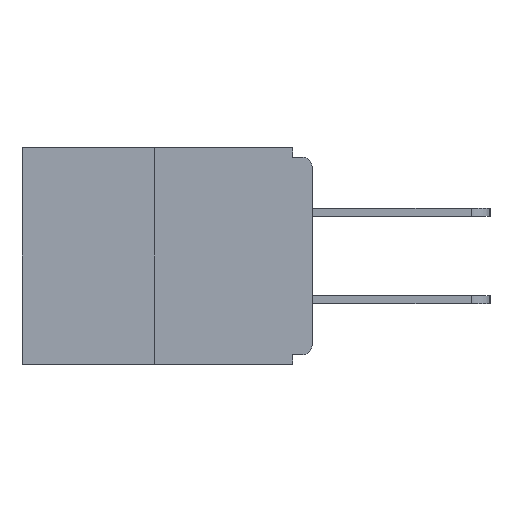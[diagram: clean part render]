
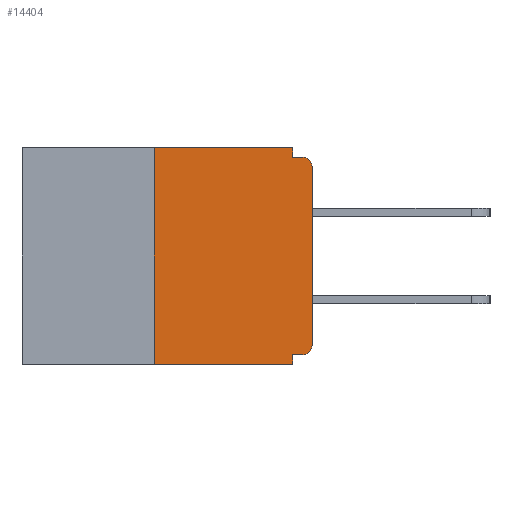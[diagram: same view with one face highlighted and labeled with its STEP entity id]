
A CAD part, left-side view. The second image highlights one B-rep face of the part: STEP entity #14404.
In plain terms, the highlighted planar face has unit normal (-1, 0, 0).
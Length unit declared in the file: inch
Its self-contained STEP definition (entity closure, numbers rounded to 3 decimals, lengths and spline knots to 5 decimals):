
#41 = LINE ( 'NONE', #24204, #22183 ) ;
#332 = DIRECTION ( 'NONE',  ( -1., 0., 0. ) ) ;
#713 = CARTESIAN_POINT ( 'NONE',  ( 0., 0.015, -0.03 ) ) ;
#792 = AXIS2_PLACEMENT_3D ( 'NONE', #713, #11689, #17690 ) ;
#1681 = VECTOR ( 'NONE', #19501, 39.37008 ) ;
#2002 = VERTEX_POINT ( 'NONE', #16268 ) ;
#2508 = PLANE ( 'NONE',  #15653 ) ;
#2662 = EDGE_CURVE ( 'NONE', #5712, #25853, #25253, .T. ) ;
#3229 = VECTOR ( 'NONE', #23539, 39.37008 ) ;
#3249 = CARTESIAN_POINT ( 'NONE',  ( 0., 0., -0.328 ) ) ;
#3826 = VECTOR ( 'NONE', #20638, 39.37008 ) ;
#4607 = LINE ( 'NONE', #23255, #6688 ) ;
#4760 = ORIENTED_EDGE ( 'NONE', *, *, #18055, .F. ) ;
#4921 = ORIENTED_EDGE ( 'NONE', *, *, #12934, .F. ) ;
#5234 = CARTESIAN_POINT ( 'NONE',  ( 0., 0.031, -0.015 ) ) ;
#5511 = FACE_OUTER_BOUND ( 'NONE', #9729, .T. ) ;
#5707 = CARTESIAN_POINT ( 'NONE',  ( 0., 0., -0.313 ) ) ;
#5712 = VERTEX_POINT ( 'NONE', #20174 ) ;
#5860 = VECTOR ( 'NONE', #27657, 39.37008 ) ;
#6462 = VERTEX_POINT ( 'NONE', #5234 ) ;
#6685 = EDGE_CURVE ( 'NONE', #16069, #20754, #12546, .T. ) ;
#6688 = VECTOR ( 'NONE', #21271, 39.37008 ) ;
#6735 = DIRECTION ( 'NONE',  ( 0., 0., -1. ) ) ;
#6820 = CARTESIAN_POINT ( 'NONE',  ( 0., 0.46, 0. ) ) ;
#6916 = DIRECTION ( 'NONE',  ( 1., 0., 0. ) ) ;
#7404 = CARTESIAN_POINT ( 'NONE',  ( 0., 0.25, 0. ) ) ;
#8445 = DIRECTION ( 'NONE',  ( 0., 0., 1. ) ) ;
#8929 = LINE ( 'NONE', #10278, #5860 ) ;
#9729 = EDGE_LOOP ( 'NONE', ( #18498, #25322, #17624, #4760, #11119, #21736, #12060, #12692, #4921, #25541 ) ) ;
#10278 = CARTESIAN_POINT ( 'NONE',  ( 0., 0.46, 0. ) ) ;
#10978 = EDGE_CURVE ( 'NONE', #5712, #16069, #27955, .T. ) ;
#11017 = VERTEX_POINT ( 'NONE', #11849 ) ;
#11119 = ORIENTED_EDGE ( 'NONE', *, *, #2662, .F. ) ;
#11344 = EDGE_CURVE ( 'NONE', #12639, #11017, #8929, .T. ) ;
#11689 = DIRECTION ( 'NONE',  ( -1., 0., 0. ) ) ;
#11849 = CARTESIAN_POINT ( 'NONE',  ( 0., 0.031, 0. ) ) ;
#11918 = EDGE_CURVE ( 'NONE', #12886, #14304, #26399, .T. ) ;
#12060 = ORIENTED_EDGE ( 'NONE', *, *, #6685, .T. ) ;
#12546 = LINE ( 'NONE', #21475, #22094 ) ;
#12639 = VERTEX_POINT ( 'NONE', #7404 ) ;
#12692 = ORIENTED_EDGE ( 'NONE', *, *, #19406, .T. ) ;
#12886 = VERTEX_POINT ( 'NONE', #19180 ) ;
#12934 = EDGE_CURVE ( 'NONE', #6462, #2002, #22286, .T. ) ;
#13142 = VECTOR ( 'NONE', #17829, 39.37008 ) ;
#13381 = CARTESIAN_POINT ( 'NONE',  ( 0., 0.015, -0.313 ) ) ;
#14304 = VERTEX_POINT ( 'NONE', #16043 ) ;
#14404 = ADVANCED_FACE ( 'NONE', ( #5511 ), #2508, .F. ) ;
#14409 = EDGE_CURVE ( 'NONE', #11017, #6462, #41, .T. ) ;
#15653 = AXIS2_PLACEMENT_3D ( 'NONE', #6820, #6916, #19647 ) ;
#16043 = CARTESIAN_POINT ( 'NONE',  ( 0., 0.031, -0.343 ) ) ;
#16069 = VERTEX_POINT ( 'NONE', #5707 ) ;
#16268 = CARTESIAN_POINT ( 'NONE',  ( 0., 0.015, -0.015 ) ) ;
#16579 = CIRCLE ( 'NONE', #792, 0.015 ) ;
#17015 = LINE ( 'NONE', #23880, #1681 ) ;
#17624 = ORIENTED_EDGE ( 'NONE', *, *, #11918, .T. ) ;
#17690 = DIRECTION ( 'NONE',  ( 0., 0., -1. ) ) ;
#17829 = DIRECTION ( 'NONE',  ( 0., -1., 0. ) ) ;
#17917 = CARTESIAN_POINT ( 'NONE',  ( 0., 0.46, -0.343 ) ) ;
#18055 = EDGE_CURVE ( 'NONE', #25853, #14304, #17015, .T. ) ;
#18498 = ORIENTED_EDGE ( 'NONE', *, *, #11344, .F. ) ;
#18526 = AXIS2_PLACEMENT_3D ( 'NONE', #13381, #332, #24308 ) ;
#19180 = CARTESIAN_POINT ( 'NONE',  ( 0., 0.25, -0.343 ) ) ;
#19406 = EDGE_CURVE ( 'NONE', #20754, #2002, #16579, .T. ) ;
#19501 = DIRECTION ( 'NONE',  ( 0., 0., -1. ) ) ;
#19647 = DIRECTION ( 'NONE',  ( 0., 0., -1. ) ) ;
#20174 = CARTESIAN_POINT ( 'NONE',  ( 0., 0.015, -0.328 ) ) ;
#20357 = CARTESIAN_POINT ( 'NONE',  ( 0., 0.031, -0.328 ) ) ;
#20638 = DIRECTION ( 'NONE',  ( 0., 1., 0. ) ) ;
#20754 = VERTEX_POINT ( 'NONE', #24160 ) ;
#21271 = DIRECTION ( 'NONE',  ( 0., 0., 1. ) ) ;
#21475 = CARTESIAN_POINT ( 'NONE',  ( 0., 0., 0. ) ) ;
#21736 = ORIENTED_EDGE ( 'NONE', *, *, #10978, .T. ) ;
#22094 = VECTOR ( 'NONE', #8445, 39.37008 ) ;
#22183 = VECTOR ( 'NONE', #6735, 39.37008 ) ;
#22286 = LINE ( 'NONE', #25724, #3229 ) ;
#23255 = CARTESIAN_POINT ( 'NONE',  ( 0., 0.25, 0. ) ) ;
#23539 = DIRECTION ( 'NONE',  ( 0., -1., 0. ) ) ;
#23880 = CARTESIAN_POINT ( 'NONE',  ( 0., 0.031, -0.343 ) ) ;
#24160 = CARTESIAN_POINT ( 'NONE',  ( 0., 0., -0.03 ) ) ;
#24204 = CARTESIAN_POINT ( 'NONE',  ( 0., 0.031, 0. ) ) ;
#24308 = DIRECTION ( 'NONE',  ( 0., 0., -1. ) ) ;
#25253 = LINE ( 'NONE', #3249, #3826 ) ;
#25322 = ORIENTED_EDGE ( 'NONE', *, *, #25436, .F. ) ;
#25436 = EDGE_CURVE ( 'NONE', #12886, #12639, #4607, .T. ) ;
#25541 = ORIENTED_EDGE ( 'NONE', *, *, #14409, .F. ) ;
#25724 = CARTESIAN_POINT ( 'NONE',  ( 0., 0., -0.015 ) ) ;
#25853 = VERTEX_POINT ( 'NONE', #20357 ) ;
#26399 = LINE ( 'NONE', #17917, #13142 ) ;
#27657 = DIRECTION ( 'NONE',  ( 0., -1., 0. ) ) ;
#27955 = CIRCLE ( 'NONE', #18526, 0.015 ) ;
